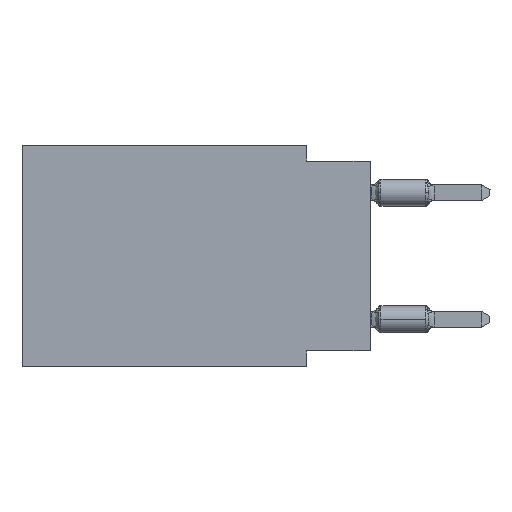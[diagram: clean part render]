
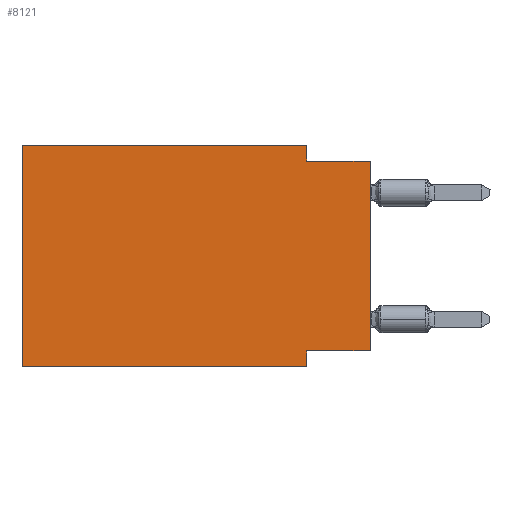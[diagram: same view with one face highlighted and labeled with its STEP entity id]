
A CAD part, left-side view. The second image highlights one B-rep face of the part: STEP entity #8121.
In plain terms, the highlighted planar face has unit normal (-1, 0, 0).
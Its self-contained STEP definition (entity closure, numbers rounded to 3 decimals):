
#539 = ORIENTED_EDGE ( 'NONE', *, *, #704, .T. ) ;
#574 = ORIENTED_EDGE ( 'NONE', *, *, #4916, .F. ) ;
#704 = EDGE_CURVE ( 'NONE', #4929, #14909, #6833, .T. ) ;
#1268 = CARTESIAN_POINT ( 'NONE',  ( 0., 2.54, -8.89 ) ) ;
#1640 = VECTOR ( 'NONE', #19924, 1000. ) ;
#1656 = DIRECTION ( 'NONE',  ( 0., 1., 0. ) ) ;
#1781 = LINE ( 'NONE', #4840, #1640 ) ;
#2431 = CARTESIAN_POINT ( 'NONE',  ( 0., 2.54, 0. ) ) ;
#3041 = CARTESIAN_POINT ( 'NONE',  ( 0., 13.97, 0. ) ) ;
#3318 = DIRECTION ( 'NONE',  ( 0., 0., 1. ) ) ;
#3436 = DIRECTION ( 'NONE',  ( 0., -1., 0. ) ) ;
#4046 = ORIENTED_EDGE ( 'NONE', *, *, #9687, .F. ) ;
#4279 = DIRECTION ( 'NONE',  ( 0., 0., -1. ) ) ;
#4302 = DIRECTION ( 'NONE',  ( 0., -1., 0. ) ) ;
#4489 = EDGE_CURVE ( 'NONE', #13068, #14909, #16682, .T. ) ;
#4492 = EDGE_CURVE ( 'NONE', #7042, #12718, #15065, .T. ) ;
#4840 = CARTESIAN_POINT ( 'NONE',  ( 0., 2.54, -8.89 ) ) ;
#4916 = EDGE_CURVE ( 'NONE', #5886, #6578, #1781, .T. ) ;
#4927 = FACE_OUTER_BOUND ( 'NONE', #14014, .T. ) ;
#4929 = VERTEX_POINT ( 'NONE', #17991 ) ;
#5728 = CARTESIAN_POINT ( 'NONE',  ( 0., 0., 0. ) ) ;
#5804 = VECTOR ( 'NONE', #4279, 1000. ) ;
#5886 = VERTEX_POINT ( 'NONE', #14981 ) ;
#6016 = LINE ( 'NONE', #2431, #5804 ) ;
#6237 = PLANE ( 'NONE',  #15698 ) ;
#6578 = VERTEX_POINT ( 'NONE', #1268 ) ;
#6833 = LINE ( 'NONE', #5728, #9441 ) ;
#6996 = LINE ( 'NONE', #18204, #9967 ) ;
#7042 = VERTEX_POINT ( 'NONE', #13708 ) ;
#7711 = CARTESIAN_POINT ( 'NONE',  ( 0., 0., -0.635 ) ) ;
#7877 = VECTOR ( 'NONE', #3436, 1000. ) ;
#8121 = ADVANCED_FACE ( 'NONE', ( #4927 ), #6237, .F. ) ;
#8700 = ORIENTED_EDGE ( 'NONE', *, *, #4489, .F. ) ;
#9144 = CARTESIAN_POINT ( 'NONE',  ( 0., 2.54, 0. ) ) ;
#9441 = VECTOR ( 'NONE', #12137, 1000. ) ;
#9687 = EDGE_CURVE ( 'NONE', #4929, #5886, #12298, .T. ) ;
#9967 = VECTOR ( 'NONE', #3318, 1000. ) ;
#10522 = ORIENTED_EDGE ( 'NONE', *, *, #19540, .F. ) ;
#11009 = VECTOR ( 'NONE', #4302, 1000. ) ;
#11356 = DIRECTION ( 'NONE',  ( 1., 0., 0. ) ) ;
#11930 = EDGE_CURVE ( 'NONE', #15692, #6578, #19073, .T. ) ;
#12137 = DIRECTION ( 'NONE',  ( 0., 0., 1. ) ) ;
#12243 = EDGE_CURVE ( 'NONE', #15692, #7042, #6996, .T. ) ;
#12298 = LINE ( 'NONE', #19580, #17730 ) ;
#12718 = VERTEX_POINT ( 'NONE', #9144 ) ;
#12922 = ORIENTED_EDGE ( 'NONE', *, *, #11930, .T. ) ;
#13068 = VERTEX_POINT ( 'NONE', #18352 ) ;
#13681 = ORIENTED_EDGE ( 'NONE', *, *, #4492, .F. ) ;
#13708 = CARTESIAN_POINT ( 'NONE',  ( 0., 13.97, 0. ) ) ;
#13762 = CARTESIAN_POINT ( 'NONE',  ( 0., 13.97, -8.89 ) ) ;
#14014 = EDGE_LOOP ( 'NONE', ( #539, #8700, #10522, #13681, #15211, #12922, #574, #4046 ) ) ;
#14116 = VECTOR ( 'NONE', #19344, 1000. ) ;
#14909 = VERTEX_POINT ( 'NONE', #15255 ) ;
#14981 = CARTESIAN_POINT ( 'NONE',  ( 0., 2.54, -8.255 ) ) ;
#15065 = LINE ( 'NONE', #3041, #14116 ) ;
#15211 = ORIENTED_EDGE ( 'NONE', *, *, #12243, .F. ) ;
#15255 = CARTESIAN_POINT ( 'NONE',  ( 0., 0., -0.635 ) ) ;
#15692 = VERTEX_POINT ( 'NONE', #13762 ) ;
#15698 = AXIS2_PLACEMENT_3D ( 'NONE', #17982, #11356, #21457 ) ;
#16682 = LINE ( 'NONE', #7711, #7877 ) ;
#17730 = VECTOR ( 'NONE', #1656, 1000. ) ;
#17982 = CARTESIAN_POINT ( 'NONE',  ( 0., 13.97, 0. ) ) ;
#17991 = CARTESIAN_POINT ( 'NONE',  ( 0., 0., -8.255 ) ) ;
#18204 = CARTESIAN_POINT ( 'NONE',  ( 0., 13.97, 0. ) ) ;
#18352 = CARTESIAN_POINT ( 'NONE',  ( 0., 2.54, -0.635 ) ) ;
#19073 = LINE ( 'NONE', #19187, #11009 ) ;
#19187 = CARTESIAN_POINT ( 'NONE',  ( 0., 13.97, -8.89 ) ) ;
#19344 = DIRECTION ( 'NONE',  ( 0., -1., 0. ) ) ;
#19540 = EDGE_CURVE ( 'NONE', #12718, #13068, #6016, .T. ) ;
#19580 = CARTESIAN_POINT ( 'NONE',  ( 0., 0., -8.255 ) ) ;
#19924 = DIRECTION ( 'NONE',  ( 0., 0., -1. ) ) ;
#21457 = DIRECTION ( 'NONE',  ( 0., 0., -1. ) ) ;
